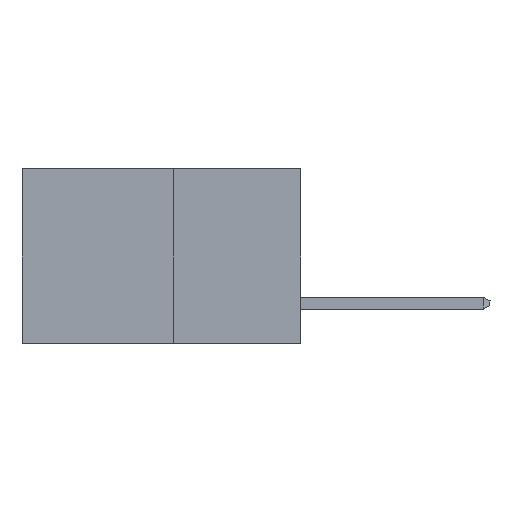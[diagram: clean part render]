
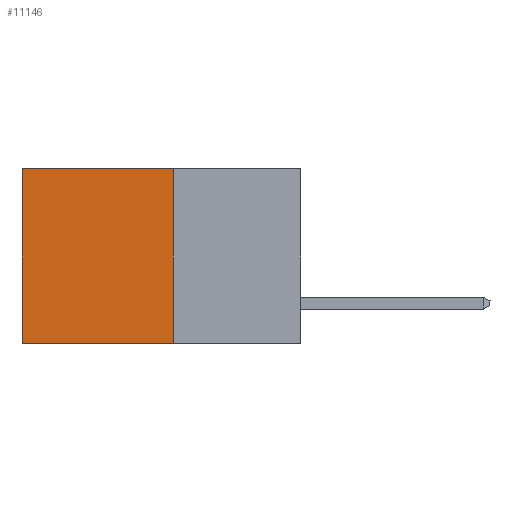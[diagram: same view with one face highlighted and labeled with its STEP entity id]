
A CAD part, left-side view. The second image highlights one B-rep face of the part: STEP entity #11146.
In plain terms, the highlighted planar face has unit normal (-1, 0, 0).
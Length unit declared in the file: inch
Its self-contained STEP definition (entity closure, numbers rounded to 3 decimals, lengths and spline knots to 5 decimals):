
#1373 = ORIENTED_EDGE ( 'NONE', *, *, #5877, .F. ) ;
#2393 = PLANE ( 'NONE',  #4492 ) ;
#3149 = VERTEX_POINT ( 'NONE', #3802 ) ;
#3802 = CARTESIAN_POINT ( 'NONE',  ( 0.277, 0.27, 0. ) ) ;
#3920 = CARTESIAN_POINT ( 'NONE',  ( 0.277, 0.27, -0.37 ) ) ;
#3978 = LINE ( 'NONE', #15062, #13594 ) ;
#4492 = AXIS2_PLACEMENT_3D ( 'NONE', #8703, #12241, #4806 ) ;
#4671 = LINE ( 'NONE', #12319, #11021 ) ;
#4806 = DIRECTION ( 'NONE',  ( 0., 0., -1. ) ) ;
#4993 = ORIENTED_EDGE ( 'NONE', *, *, #12077, .T. ) ;
#5877 = EDGE_CURVE ( 'NONE', #8151, #8619, #3978, .T. ) ;
#6208 = DIRECTION ( 'NONE',  ( 0., 1., 0. ) ) ;
#6509 = CARTESIAN_POINT ( 'NONE',  ( 0.277, 0.59, -0.37 ) ) ;
#6784 = VERTEX_POINT ( 'NONE', #11709 ) ;
#7087 = LINE ( 'NONE', #6509, #13028 ) ;
#7697 = ORIENTED_EDGE ( 'NONE', *, *, #13958, .T. ) ;
#8151 = VERTEX_POINT ( 'NONE', #3920 ) ;
#8619 = VERTEX_POINT ( 'NONE', #14625 ) ;
#8681 = VECTOR ( 'NONE', #12333, 39.37008 ) ;
#8703 = CARTESIAN_POINT ( 'NONE',  ( 0.277, 0.27, -0.37 ) ) ;
#9603 = DIRECTION ( 'NONE',  ( 0., 1., 0. ) ) ;
#10319 = DIRECTION ( 'NONE',  ( 0., 0., -1. ) ) ;
#10783 = LINE ( 'NONE', #11276, #8681 ) ;
#11021 = VECTOR ( 'NONE', #6208, 39.37008 ) ;
#11146 = ADVANCED_FACE ( 'NONE', ( #13929 ), #2393, .F. ) ;
#11276 = CARTESIAN_POINT ( 'NONE',  ( 0.277, 0.27, -0.37 ) ) ;
#11709 = CARTESIAN_POINT ( 'NONE',  ( 0.277, 0.59, 0. ) ) ;
#12077 = EDGE_CURVE ( 'NONE', #3149, #6784, #4671, .T. ) ;
#12241 = DIRECTION ( 'NONE',  ( 1., 0., 0. ) ) ;
#12319 = CARTESIAN_POINT ( 'NONE',  ( 0.277, 0.27, 0. ) ) ;
#12333 = DIRECTION ( 'NONE',  ( 0., 0., -1. ) ) ;
#13028 = VECTOR ( 'NONE', #10319, 39.37008 ) ;
#13594 = VECTOR ( 'NONE', #9603, 39.37008 ) ;
#13929 = FACE_OUTER_BOUND ( 'NONE', #15050, .T. ) ;
#13958 = EDGE_CURVE ( 'NONE', #6784, #8619, #7087, .T. ) ;
#14184 = ORIENTED_EDGE ( 'NONE', *, *, #15125, .F. ) ;
#14625 = CARTESIAN_POINT ( 'NONE',  ( 0.277, 0.59, -0.37 ) ) ;
#15050 = EDGE_LOOP ( 'NONE', ( #7697, #1373, #14184, #4993 ) ) ;
#15062 = CARTESIAN_POINT ( 'NONE',  ( 0.277, 0.27, -0.37 ) ) ;
#15125 = EDGE_CURVE ( 'NONE', #3149, #8151, #10783, .T. ) ;
